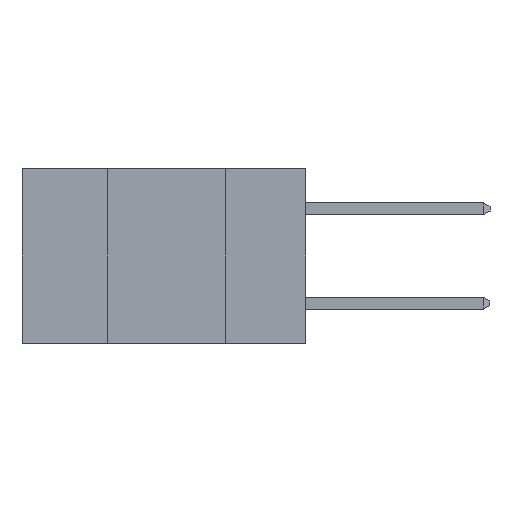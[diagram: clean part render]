
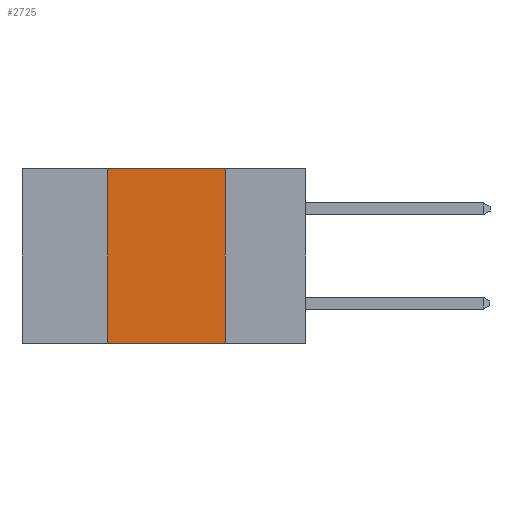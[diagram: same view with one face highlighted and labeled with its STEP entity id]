
A CAD part, left-side view. The second image highlights one B-rep face of the part: STEP entity #2725.
In plain terms, the highlighted planar face has unit normal (-1, 0, 0).
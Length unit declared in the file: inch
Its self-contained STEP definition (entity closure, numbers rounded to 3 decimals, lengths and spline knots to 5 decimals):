
#1706 = EDGE_CURVE ( 'NONE', #14023, #17147, #28566, .T. ) ;
#2555 = CARTESIAN_POINT ( 'NONE',  ( 0., 0.17, 0. ) ) ;
#2604 = LINE ( 'NONE', #4878, #20005 ) ;
#2725 = ADVANCED_FACE ( 'NONE', ( #6865 ), #12914, .F. ) ;
#4205 = EDGE_CURVE ( 'NONE', #9555, #25392, #27410, .T. ) ;
#4878 = CARTESIAN_POINT ( 'NONE',  ( 0., 0.6, 0. ) ) ;
#5899 = LINE ( 'NONE', #11463, #11237 ) ;
#6865 = FACE_OUTER_BOUND ( 'NONE', #7459, .T. ) ;
#7128 = DIRECTION ( 'NONE',  ( 0., -1., 0. ) ) ;
#7327 = EDGE_CURVE ( 'NONE', #25392, #14023, #2604, .T. ) ;
#7459 = EDGE_LOOP ( 'NONE', ( #11946, #19428, #25438, #20836 ) ) ;
#8588 = CARTESIAN_POINT ( 'NONE',  ( 0., 0.42, -0.37 ) ) ;
#8654 = AXIS2_PLACEMENT_3D ( 'NONE', #19656, #18182, #18091 ) ;
#8773 = DIRECTION ( 'NONE',  ( 0., 0., 1. ) ) ;
#9180 = DIRECTION ( 'NONE',  ( 0., -1., 0. ) ) ;
#9299 = VECTOR ( 'NONE', #8773, 39.37008 ) ;
#9555 = VERTEX_POINT ( 'NONE', #8588 ) ;
#11237 = VECTOR ( 'NONE', #9180, 39.37008 ) ;
#11463 = CARTESIAN_POINT ( 'NONE',  ( 0., 0.6, -0.37 ) ) ;
#11946 = ORIENTED_EDGE ( 'NONE', *, *, #1706, .F. ) ;
#12914 = PLANE ( 'NONE',  #8654 ) ;
#14023 = VERTEX_POINT ( 'NONE', #2555 ) ;
#16170 = DIRECTION ( 'NONE',  ( 0., 0., -1. ) ) ;
#16602 = VECTOR ( 'NONE', #16170, 39.37008 ) ;
#17147 = VERTEX_POINT ( 'NONE', #26019 ) ;
#18091 = DIRECTION ( 'NONE',  ( 0., 0., -1. ) ) ;
#18182 = DIRECTION ( 'NONE',  ( 1., 0., 0. ) ) ;
#19428 = ORIENTED_EDGE ( 'NONE', *, *, #7327, .F. ) ;
#19656 = CARTESIAN_POINT ( 'NONE',  ( 0., 0.6, 0. ) ) ;
#20005 = VECTOR ( 'NONE', #7128, 39.37008 ) ;
#20836 = ORIENTED_EDGE ( 'NONE', *, *, #26186, .T. ) ;
#23393 = CARTESIAN_POINT ( 'NONE',  ( 0., 0.17, 0. ) ) ;
#25392 = VERTEX_POINT ( 'NONE', #27082 ) ;
#25438 = ORIENTED_EDGE ( 'NONE', *, *, #4205, .F. ) ;
#25755 = CARTESIAN_POINT ( 'NONE',  ( 0., 0.42, 0. ) ) ;
#26019 = CARTESIAN_POINT ( 'NONE',  ( 0., 0.17, -0.37 ) ) ;
#26186 = EDGE_CURVE ( 'NONE', #9555, #17147, #5899, .T. ) ;
#27082 = CARTESIAN_POINT ( 'NONE',  ( 0., 0.42, 0. ) ) ;
#27410 = LINE ( 'NONE', #25755, #9299 ) ;
#28566 = LINE ( 'NONE', #23393, #16602 ) ;
